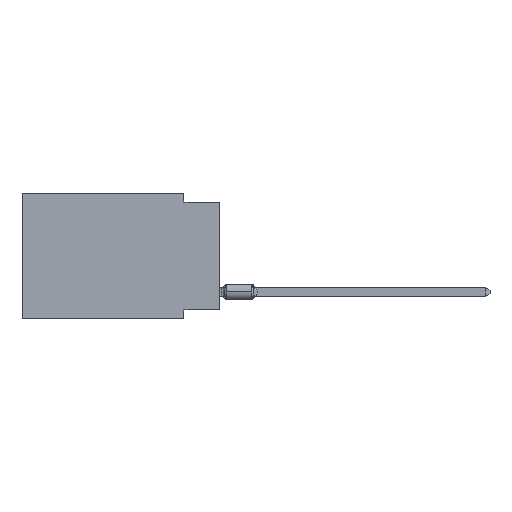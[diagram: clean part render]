
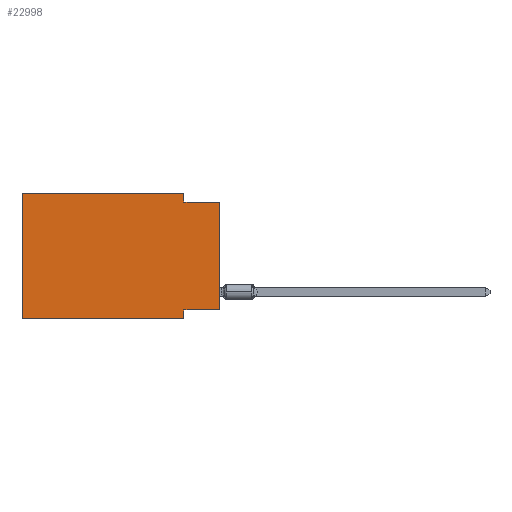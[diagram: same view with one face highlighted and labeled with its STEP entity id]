
A CAD part, left-side view. The second image highlights one B-rep face of the part: STEP entity #22998.
In plain terms, the highlighted planar face has unit normal (-1, 0, 0).
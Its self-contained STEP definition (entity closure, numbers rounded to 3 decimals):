
#518 = CARTESIAN_POINT ( 'NONE',  ( 0., 2.54, 0. ) ) ;
#716 = CARTESIAN_POINT ( 'NONE',  ( 0., 0., -8.255 ) ) ;
#786 = VERTEX_POINT ( 'NONE', #23585 ) ;
#1220 = VERTEX_POINT ( 'NONE', #6502 ) ;
#1694 = LINE ( 'NONE', #30667, #19250 ) ;
#3460 = VERTEX_POINT ( 'NONE', #518 ) ;
#3774 = ORIENTED_EDGE ( 'NONE', *, *, #18094, .F. ) ;
#4155 = LINE ( 'NONE', #13853, #22713 ) ;
#4210 = VERTEX_POINT ( 'NONE', #716 ) ;
#4328 = DIRECTION ( 'NONE',  ( 0., 1., 0. ) ) ;
#5063 = AXIS2_PLACEMENT_3D ( 'NONE', #16719, #25981, #6715 ) ;
#6502 = CARTESIAN_POINT ( 'NONE',  ( 0., 2.54, -8.255 ) ) ;
#6715 = DIRECTION ( 'NONE',  ( 0., 0., -1. ) ) ;
#7145 = ORIENTED_EDGE ( 'NONE', *, *, #22607, .F. ) ;
#7190 = EDGE_LOOP ( 'NONE', ( #24811, #30979, #16850, #24656, #23936, #11870, #7145, #3774 ) ) ;
#7912 = LINE ( 'NONE', #10131, #21928 ) ;
#8984 = VERTEX_POINT ( 'NONE', #24153 ) ;
#9950 = EDGE_CURVE ( 'NONE', #28613, #3460, #12737, .T. ) ;
#10024 = VECTOR ( 'NONE', #25049, 1000. ) ;
#10131 = CARTESIAN_POINT ( 'NONE',  ( 0., 0., -0.635 ) ) ;
#10484 = CARTESIAN_POINT ( 'NONE',  ( 0., 13.97, -8.89 ) ) ;
#10710 = EDGE_CURVE ( 'NONE', #21158, #8984, #4155, .T. ) ;
#11223 = LINE ( 'NONE', #30505, #21420 ) ;
#11331 = LINE ( 'NONE', #16438, #31161 ) ;
#11695 = EDGE_CURVE ( 'NONE', #3460, #29641, #20083, .T. ) ;
#11870 = ORIENTED_EDGE ( 'NONE', *, *, #10710, .T. ) ;
#12737 = LINE ( 'NONE', #13207, #14111 ) ;
#13207 = CARTESIAN_POINT ( 'NONE',  ( 0., 13.97, 0. ) ) ;
#13610 = DIRECTION ( 'NONE',  ( 0., 0., -1. ) ) ;
#13853 = CARTESIAN_POINT ( 'NONE',  ( 0., 13.97, -8.89 ) ) ;
#14111 = VECTOR ( 'NONE', #22461, 1000. ) ;
#14705 = VECTOR ( 'NONE', #27369, 1000. ) ;
#15233 = DIRECTION ( 'NONE',  ( 0., -1., 0. ) ) ;
#16273 = EDGE_CURVE ( 'NONE', #29641, #786, #7912, .T. ) ;
#16438 = CARTESIAN_POINT ( 'NONE',  ( 0., 0., -8.255 ) ) ;
#16515 = EDGE_CURVE ( 'NONE', #4210, #786, #11223, .T. ) ;
#16698 = CARTESIAN_POINT ( 'NONE',  ( 0., 2.54, -0.635 ) ) ;
#16719 = CARTESIAN_POINT ( 'NONE',  ( 0., 13.97, 0. ) ) ;
#16850 = ORIENTED_EDGE ( 'NONE', *, *, #11695, .F. ) ;
#18016 = CARTESIAN_POINT ( 'NONE',  ( 0., 2.54, 0. ) ) ;
#18094 = EDGE_CURVE ( 'NONE', #4210, #1220, #11331, .T. ) ;
#19250 = VECTOR ( 'NONE', #13610, 1000. ) ;
#20083 = LINE ( 'NONE', #18016, #10024 ) ;
#20510 = CARTESIAN_POINT ( 'NONE',  ( 0., 13.97, 0. ) ) ;
#21158 = VERTEX_POINT ( 'NONE', #10484 ) ;
#21420 = VECTOR ( 'NONE', #28256, 1000. ) ;
#21928 = VECTOR ( 'NONE', #15233, 1000. ) ;
#22446 = LINE ( 'NONE', #20510, #14705 ) ;
#22461 = DIRECTION ( 'NONE',  ( 0., -1., 0. ) ) ;
#22607 = EDGE_CURVE ( 'NONE', #1220, #8984, #1694, .T. ) ;
#22713 = VECTOR ( 'NONE', #30426, 1000. ) ;
#22998 = ADVANCED_FACE ( 'NONE', ( #28993 ), #25811, .F. ) ;
#23585 = CARTESIAN_POINT ( 'NONE',  ( 0., 0., -0.635 ) ) ;
#23936 = ORIENTED_EDGE ( 'NONE', *, *, #29765, .F. ) ;
#24153 = CARTESIAN_POINT ( 'NONE',  ( 0., 2.54, -8.89 ) ) ;
#24656 = ORIENTED_EDGE ( 'NONE', *, *, #9950, .F. ) ;
#24811 = ORIENTED_EDGE ( 'NONE', *, *, #16515, .T. ) ;
#25049 = DIRECTION ( 'NONE',  ( 0., 0., -1. ) ) ;
#25146 = CARTESIAN_POINT ( 'NONE',  ( 0., 13.97, 0. ) ) ;
#25811 = PLANE ( 'NONE',  #5063 ) ;
#25981 = DIRECTION ( 'NONE',  ( 1., 0., 0. ) ) ;
#27369 = DIRECTION ( 'NONE',  ( 0., 0., 1. ) ) ;
#28256 = DIRECTION ( 'NONE',  ( 0., 0., 1. ) ) ;
#28613 = VERTEX_POINT ( 'NONE', #25146 ) ;
#28993 = FACE_OUTER_BOUND ( 'NONE', #7190, .T. ) ;
#29641 = VERTEX_POINT ( 'NONE', #16698 ) ;
#29765 = EDGE_CURVE ( 'NONE', #21158, #28613, #22446, .T. ) ;
#30426 = DIRECTION ( 'NONE',  ( 0., -1., 0. ) ) ;
#30505 = CARTESIAN_POINT ( 'NONE',  ( 0., 0., 0. ) ) ;
#30667 = CARTESIAN_POINT ( 'NONE',  ( 0., 2.54, -8.89 ) ) ;
#30979 = ORIENTED_EDGE ( 'NONE', *, *, #16273, .F. ) ;
#31161 = VECTOR ( 'NONE', #4328, 1000. ) ;
